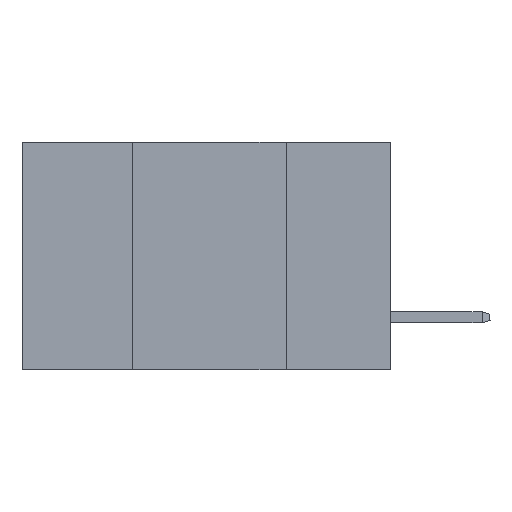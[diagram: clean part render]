
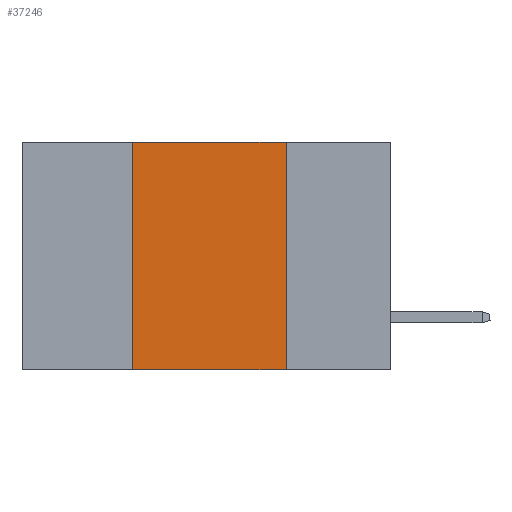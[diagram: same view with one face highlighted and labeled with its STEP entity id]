
A CAD part, left-side view. The second image highlights one B-rep face of the part: STEP entity #37246.
In plain terms, the highlighted planar face has unit normal (-1, 0, 0).
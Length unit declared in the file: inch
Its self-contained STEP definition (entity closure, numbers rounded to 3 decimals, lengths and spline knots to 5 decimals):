
#1008 = DIRECTION ( 'NONE',  ( 0., -1., 0. ) ) ;
#1399 = CARTESIAN_POINT ( 'NONE',  ( 0., 0.17, -0.37 ) ) ;
#1598 = VERTEX_POINT ( 'NONE', #1399 ) ;
#2393 = VERTEX_POINT ( 'NONE', #6857 ) ;
#4024 = DIRECTION ( 'NONE',  ( 0., 0., -1. ) ) ;
#4354 = DIRECTION ( 'NONE',  ( 0., 0., -1. ) ) ;
#4508 = EDGE_LOOP ( 'NONE', ( #15215, #16375, #19363, #26482 ) ) ;
#5851 = EDGE_CURVE ( 'NONE', #20633, #2393, #11297, .T. ) ;
#6279 = CARTESIAN_POINT ( 'NONE',  ( 0., 0.42, 0. ) ) ;
#6857 = CARTESIAN_POINT ( 'NONE',  ( 0., 0.17, 0. ) ) ;
#7998 = LINE ( 'NONE', #25028, #23502 ) ;
#8551 = FACE_OUTER_BOUND ( 'NONE', #4508, .T. ) ;
#11297 = LINE ( 'NONE', #14706, #17697 ) ;
#14632 = CARTESIAN_POINT ( 'NONE',  ( 0., 0.6, 0. ) ) ;
#14706 = CARTESIAN_POINT ( 'NONE',  ( 0., 0.6, 0. ) ) ;
#15215 = ORIENTED_EDGE ( 'NONE', *, *, #36695, .F. ) ;
#16375 = ORIENTED_EDGE ( 'NONE', *, *, #5851, .F. ) ;
#17621 = PLANE ( 'NONE',  #26474 ) ;
#17697 = VECTOR ( 'NONE', #32945, 39.37008 ) ;
#19363 = ORIENTED_EDGE ( 'NONE', *, *, #32343, .F. ) ;
#20633 = VERTEX_POINT ( 'NONE', #36955 ) ;
#22074 = CARTESIAN_POINT ( 'NONE',  ( 0., 0.6, -0.37 ) ) ;
#23502 = VECTOR ( 'NONE', #4024, 39.37008 ) ;
#24850 = VECTOR ( 'NONE', #1008, 39.37008 ) ;
#25028 = CARTESIAN_POINT ( 'NONE',  ( 0., 0.17, 0. ) ) ;
#25989 = LINE ( 'NONE', #22074, #24850 ) ;
#26474 = AXIS2_PLACEMENT_3D ( 'NONE', #14632, #35104, #4354 ) ;
#26482 = ORIENTED_EDGE ( 'NONE', *, *, #38320, .T. ) ;
#28786 = CARTESIAN_POINT ( 'NONE',  ( 0., 0.42, -0.37 ) ) ;
#31423 = VECTOR ( 'NONE', #40681, 39.37008 ) ;
#32343 = EDGE_CURVE ( 'NONE', #33940, #20633, #42103, .T. ) ;
#32945 = DIRECTION ( 'NONE',  ( 0., -1., 0. ) ) ;
#33940 = VERTEX_POINT ( 'NONE', #28786 ) ;
#35104 = DIRECTION ( 'NONE',  ( 1., 0., 0. ) ) ;
#36695 = EDGE_CURVE ( 'NONE', #2393, #1598, #7998, .T. ) ;
#36955 = CARTESIAN_POINT ( 'NONE',  ( 0., 0.42, 0. ) ) ;
#37246 = ADVANCED_FACE ( 'NONE', ( #8551 ), #17621, .F. ) ;
#38320 = EDGE_CURVE ( 'NONE', #33940, #1598, #25989, .T. ) ;
#40681 = DIRECTION ( 'NONE',  ( 0., 0., 1. ) ) ;
#42103 = LINE ( 'NONE', #6279, #31423 ) ;
